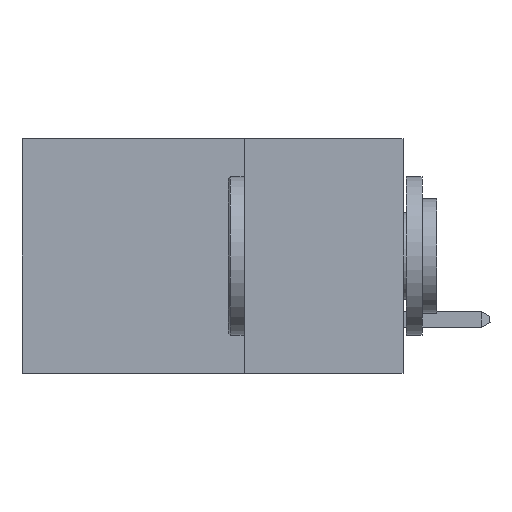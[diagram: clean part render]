
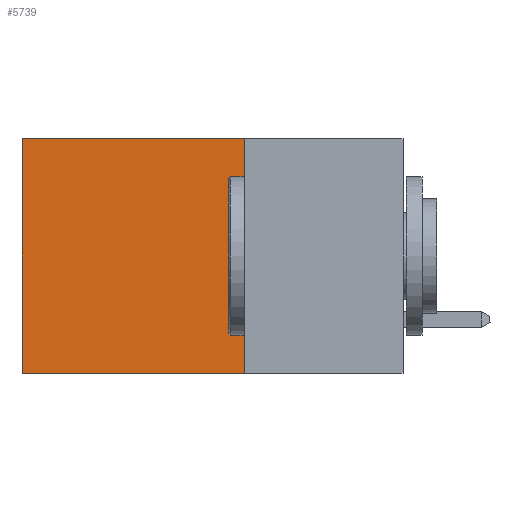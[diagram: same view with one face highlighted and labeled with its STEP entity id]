
A CAD part, left-side view. The second image highlights one B-rep face of the part: STEP entity #5739.
In plain terms, the highlighted planar face has unit normal (-1, 0, 0).
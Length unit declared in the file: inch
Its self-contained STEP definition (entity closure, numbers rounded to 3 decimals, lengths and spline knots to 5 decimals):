
#44 = VERTEX_POINT ( 'NONE', #8364 ) ;
#1159 = CARTESIAN_POINT ( 'NONE',  ( 0.2875, 0.25, 0. ) ) ;
#1291 = EDGE_CURVE ( 'NONE', #5194, #40608, #23351, .T. ) ;
#2363 = EDGE_CURVE ( 'NONE', #32402, #40608, #2531, .T. ) ;
#2531 = LINE ( 'NONE', #43041, #13766 ) ;
#4019 = DIRECTION ( 'NONE',  ( 0., 0., -1. ) ) ;
#4556 = EDGE_CURVE ( 'NONE', #44, #5194, #30355, .T. ) ;
#5194 = VERTEX_POINT ( 'NONE', #34507 ) ;
#5739 = ADVANCED_FACE ( 'NONE', ( #35248 ), #22843, .F. ) ;
#7051 = AXIS2_PLACEMENT_3D ( 'NONE', #41801, #26615, #4019 ) ;
#8364 = CARTESIAN_POINT ( 'NONE',  ( 0.2875, 0.25, 0. ) ) ;
#9597 = LINE ( 'NONE', #16830, #35538 ) ;
#10257 = CARTESIAN_POINT ( 'NONE',  ( 0.2875, 0.6, 0. ) ) ;
#10724 = EDGE_LOOP ( 'NONE', ( #46958, #32604, #44226, #18501 ) ) ;
#11212 = VECTOR ( 'NONE', #24100, 39.37008 ) ;
#13050 = CARTESIAN_POINT ( 'NONE',  ( 0.2875, 0.25, -0.37 ) ) ;
#13766 = VECTOR ( 'NONE', #39393, 39.37008 ) ;
#16830 = CARTESIAN_POINT ( 'NONE',  ( 0.2875, 0.25, 0. ) ) ;
#18501 = ORIENTED_EDGE ( 'NONE', *, *, #4556, .T. ) ;
#22718 = VECTOR ( 'NONE', #32446, 39.37008 ) ;
#22843 = PLANE ( 'NONE',  #7051 ) ;
#23351 = LINE ( 'NONE', #10257, #22718 ) ;
#24100 = DIRECTION ( 'NONE',  ( 0., 1., 0. ) ) ;
#25365 = CARTESIAN_POINT ( 'NONE',  ( 0.2875, 0.6, -0.37 ) ) ;
#26615 = DIRECTION ( 'NONE',  ( 1., 0., 0. ) ) ;
#30355 = LINE ( 'NONE', #1159, #11212 ) ;
#32402 = VERTEX_POINT ( 'NONE', #13050 ) ;
#32446 = DIRECTION ( 'NONE',  ( 0., 0., -1. ) ) ;
#32604 = ORIENTED_EDGE ( 'NONE', *, *, #2363, .F. ) ;
#34507 = CARTESIAN_POINT ( 'NONE',  ( 0.2875, 0.6, 0. ) ) ;
#35248 = FACE_OUTER_BOUND ( 'NONE', #10724, .T. ) ;
#35538 = VECTOR ( 'NONE', #39877, 39.37008 ) ;
#35899 = EDGE_CURVE ( 'NONE', #44, #32402, #9597, .T. ) ;
#39393 = DIRECTION ( 'NONE',  ( 0., 1., 0. ) ) ;
#39877 = DIRECTION ( 'NONE',  ( 0., 0., -1. ) ) ;
#40608 = VERTEX_POINT ( 'NONE', #25365 ) ;
#41801 = CARTESIAN_POINT ( 'NONE',  ( 0.2875, 0.25, 0. ) ) ;
#43041 = CARTESIAN_POINT ( 'NONE',  ( 0.2875, 0.25, -0.37 ) ) ;
#44226 = ORIENTED_EDGE ( 'NONE', *, *, #35899, .F. ) ;
#46958 = ORIENTED_EDGE ( 'NONE', *, *, #1291, .T. ) ;
